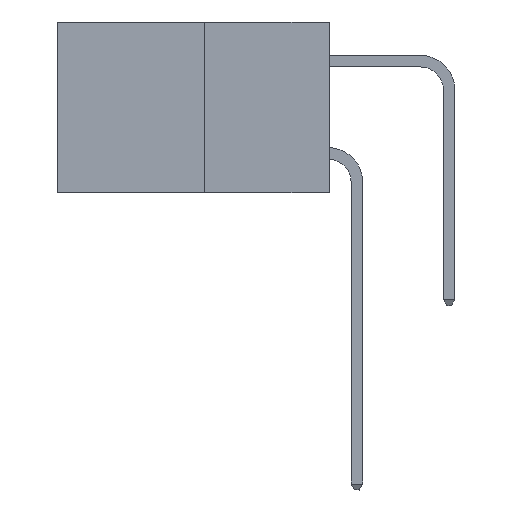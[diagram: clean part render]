
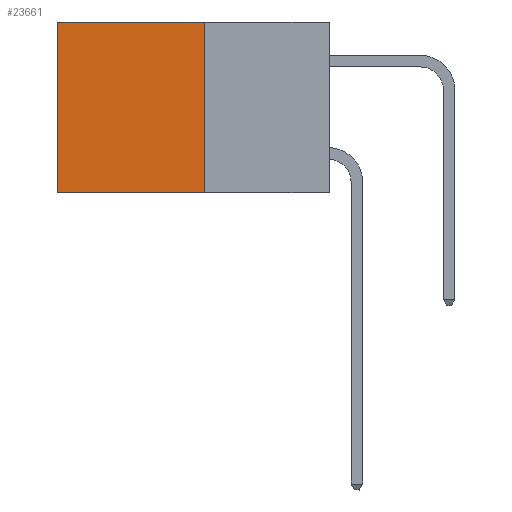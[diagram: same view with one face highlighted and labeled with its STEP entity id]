
A CAD part, left-side view. The second image highlights one B-rep face of the part: STEP entity #23661.
In plain terms, the highlighted planar face has unit normal (-1, 0, 0).
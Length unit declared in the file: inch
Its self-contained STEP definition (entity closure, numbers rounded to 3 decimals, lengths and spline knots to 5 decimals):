
#1120 = CARTESIAN_POINT ( 'NONE',  ( 0.277, 0.27, 0. ) ) ;
#1515 = EDGE_CURVE ( 'NONE', #16247, #29048, #28927, .T. ) ;
#4206 = VECTOR ( 'NONE', #29757, 39.37008 ) ;
#4946 = LINE ( 'NONE', #27390, #4206 ) ;
#5905 = ORIENTED_EDGE ( 'NONE', *, *, #13462, .F. ) ;
#6676 = CARTESIAN_POINT ( 'NONE',  ( 0.277, 0.27, -0.37 ) ) ;
#7369 = LINE ( 'NONE', #17910, #25685 ) ;
#8934 = PLANE ( 'NONE',  #29606 ) ;
#9037 = DIRECTION ( 'NONE',  ( 1., 0., 0. ) ) ;
#10764 = CARTESIAN_POINT ( 'NONE',  ( 0.277, 0.27, 0. ) ) ;
#13462 = EDGE_CURVE ( 'NONE', #16247, #23392, #7369, .T. ) ;
#14103 = LINE ( 'NONE', #16423, #27522 ) ;
#14181 = VERTEX_POINT ( 'NONE', #29637 ) ;
#15974 = ORIENTED_EDGE ( 'NONE', *, *, #16996, .F. ) ;
#16247 = VERTEX_POINT ( 'NONE', #1120 ) ;
#16423 = CARTESIAN_POINT ( 'NONE',  ( 0.277, 0.59, -0.37 ) ) ;
#16996 = EDGE_CURVE ( 'NONE', #23392, #14181, #4946, .T. ) ;
#17450 = CARTESIAN_POINT ( 'NONE',  ( 0.277, 0.59, 0. ) ) ;
#17824 = CARTESIAN_POINT ( 'NONE',  ( 0.277, 0.27, -0.37 ) ) ;
#17910 = CARTESIAN_POINT ( 'NONE',  ( 0.277, 0.27, -0.37 ) ) ;
#18923 = EDGE_LOOP ( 'NONE', ( #29956, #15974, #5905, #26353 ) ) ;
#20300 = DIRECTION ( 'NONE',  ( 0., 0., -1. ) ) ;
#21943 = VECTOR ( 'NONE', #22730, 39.37008 ) ;
#22730 = DIRECTION ( 'NONE',  ( 0., 1., 0. ) ) ;
#23392 = VERTEX_POINT ( 'NONE', #17824 ) ;
#23520 = DIRECTION ( 'NONE',  ( 0., 0., -1. ) ) ;
#23661 = ADVANCED_FACE ( 'NONE', ( #29392 ), #8934, .F. ) ;
#25339 = EDGE_CURVE ( 'NONE', #29048, #14181, #14103, .T. ) ;
#25685 = VECTOR ( 'NONE', #20300, 39.37008 ) ;
#25798 = DIRECTION ( 'NONE',  ( 0., 0., -1. ) ) ;
#26353 = ORIENTED_EDGE ( 'NONE', *, *, #1515, .T. ) ;
#27390 = CARTESIAN_POINT ( 'NONE',  ( 0.277, 0.27, -0.37 ) ) ;
#27522 = VECTOR ( 'NONE', #23520, 39.37008 ) ;
#28927 = LINE ( 'NONE', #10764, #21943 ) ;
#29048 = VERTEX_POINT ( 'NONE', #17450 ) ;
#29392 = FACE_OUTER_BOUND ( 'NONE', #18923, .T. ) ;
#29606 = AXIS2_PLACEMENT_3D ( 'NONE', #6676, #9037, #25798 ) ;
#29637 = CARTESIAN_POINT ( 'NONE',  ( 0.277, 0.59, -0.37 ) ) ;
#29757 = DIRECTION ( 'NONE',  ( 0., 1., 0. ) ) ;
#29956 = ORIENTED_EDGE ( 'NONE', *, *, #25339, .T. ) ;
